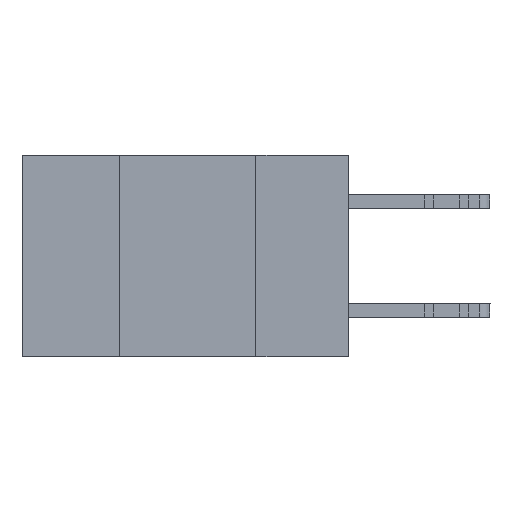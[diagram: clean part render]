
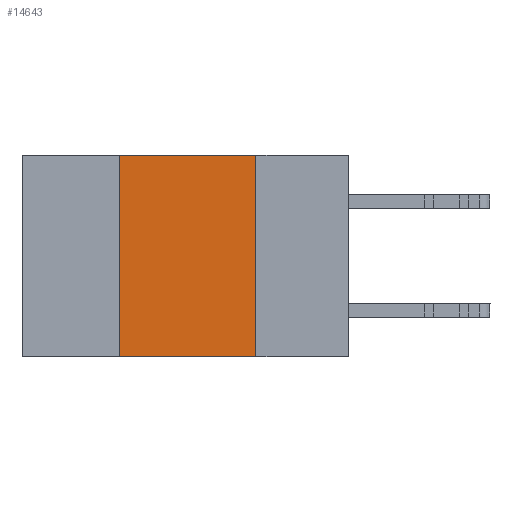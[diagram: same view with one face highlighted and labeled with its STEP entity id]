
A CAD part, left-side view. The second image highlights one B-rep face of the part: STEP entity #14643.
In plain terms, the highlighted planar face has unit normal (-1, 0, 0).
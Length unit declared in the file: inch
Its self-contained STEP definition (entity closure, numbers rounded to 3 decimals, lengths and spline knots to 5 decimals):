
#734 = AXIS2_PLACEMENT_3D ( 'NONE', #3647, #18510, #7431 ) ;
#1575 = CARTESIAN_POINT ( 'NONE',  ( 0., 0.17, 0. ) ) ;
#2993 = VERTEX_POINT ( 'NONE', #1575 ) ;
#3424 = LINE ( 'NONE', #19133, #17687 ) ;
#3505 = EDGE_CURVE ( 'NONE', #14799, #6727, #3424, .T. ) ;
#3647 = CARTESIAN_POINT ( 'NONE',  ( 0., 0.6, 0. ) ) ;
#4391 = EDGE_LOOP ( 'NONE', ( #16501, #11841, #6975, #21166 ) ) ;
#5459 = LINE ( 'NONE', #15148, #19658 ) ;
#5468 = LINE ( 'NONE', #14757, #23918 ) ;
#5819 = CARTESIAN_POINT ( 'NONE',  ( 0., 0.17, -0.37 ) ) ;
#6030 = DIRECTION ( 'NONE',  ( 0., -1., 0. ) ) ;
#6727 = VERTEX_POINT ( 'NONE', #12314 ) ;
#6975 = ORIENTED_EDGE ( 'NONE', *, *, #3505, .F. ) ;
#7431 = DIRECTION ( 'NONE',  ( 0., 0., -1. ) ) ;
#7680 = DIRECTION ( 'NONE',  ( 0., 0., -1. ) ) ;
#8031 = EDGE_CURVE ( 'NONE', #6727, #2993, #5459, .T. ) ;
#10401 = LINE ( 'NONE', #5819, #19681 ) ;
#11841 = ORIENTED_EDGE ( 'NONE', *, *, #8031, .F. ) ;
#12314 = CARTESIAN_POINT ( 'NONE',  ( 0., 0.42, 0. ) ) ;
#12954 = EDGE_CURVE ( 'NONE', #2993, #23255, #10401, .T. ) ;
#14643 = ADVANCED_FACE ( 'NONE', ( #17323 ), #20300, .F. ) ;
#14757 = CARTESIAN_POINT ( 'NONE',  ( 0., 0.6, -0.37 ) ) ;
#14799 = VERTEX_POINT ( 'NONE', #18903 ) ;
#15148 = CARTESIAN_POINT ( 'NONE',  ( 0., 0.6, 0. ) ) ;
#16501 = ORIENTED_EDGE ( 'NONE', *, *, #12954, .F. ) ;
#17323 = FACE_OUTER_BOUND ( 'NONE', #4391, .T. ) ;
#17354 = DIRECTION ( 'NONE',  ( 0., 0., 1. ) ) ;
#17687 = VECTOR ( 'NONE', #17354, 39.37008 ) ;
#18510 = DIRECTION ( 'NONE',  ( 1., 0., 0. ) ) ;
#18903 = CARTESIAN_POINT ( 'NONE',  ( 0., 0.42, -0.37 ) ) ;
#19133 = CARTESIAN_POINT ( 'NONE',  ( 0., 0.42, -0.37 ) ) ;
#19214 = EDGE_CURVE ( 'NONE', #14799, #23255, #5468, .T. ) ;
#19658 = VECTOR ( 'NONE', #6030, 39.37008 ) ;
#19681 = VECTOR ( 'NONE', #7680, 39.37008 ) ;
#20300 = PLANE ( 'NONE',  #734 ) ;
#21166 = ORIENTED_EDGE ( 'NONE', *, *, #19214, .T. ) ;
#22664 = CARTESIAN_POINT ( 'NONE',  ( 0., 0.17, -0.37 ) ) ;
#23255 = VERTEX_POINT ( 'NONE', #22664 ) ;
#23918 = VECTOR ( 'NONE', #23932, 39.37008 ) ;
#23932 = DIRECTION ( 'NONE',  ( 0., -1., 0. ) ) ;
